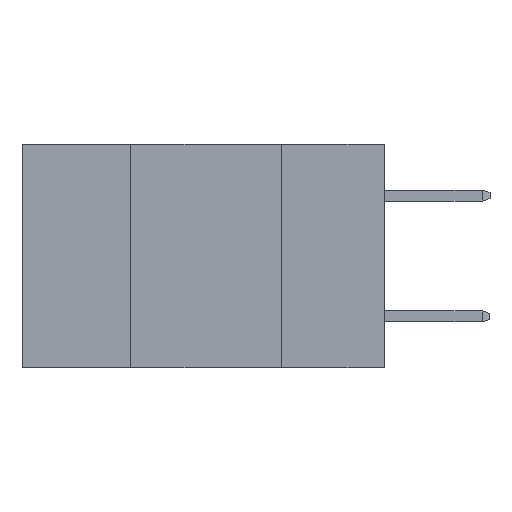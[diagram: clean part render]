
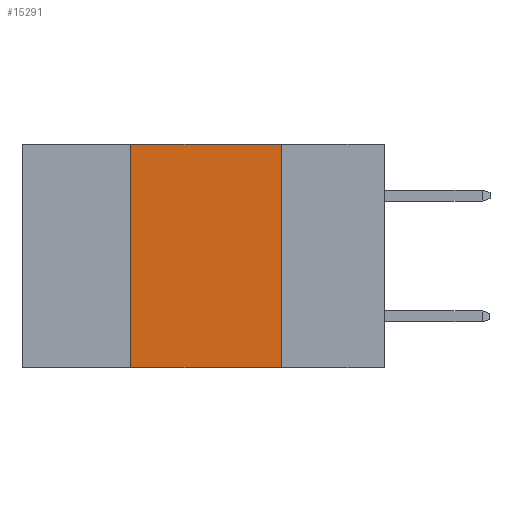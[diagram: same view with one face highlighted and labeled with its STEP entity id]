
A CAD part, left-side view. The second image highlights one B-rep face of the part: STEP entity #15291.
In plain terms, the highlighted planar face has unit normal (-1, 0, 0).
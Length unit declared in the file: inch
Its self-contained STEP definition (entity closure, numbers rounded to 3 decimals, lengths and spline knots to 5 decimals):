
#799 = EDGE_CURVE ( 'NONE', #2177, #25456, #13775, .T. ) ;
#2110 = CARTESIAN_POINT ( 'NONE',  ( 0., 0.42, 0. ) ) ;
#2177 = VERTEX_POINT ( 'NONE', #5522 ) ;
#2531 = PLANE ( 'NONE',  #17912 ) ;
#3132 = VERTEX_POINT ( 'NONE', #2110 ) ;
#3241 = EDGE_LOOP ( 'NONE', ( #24996, #9982, #10603, #21034 ) ) ;
#5432 = LINE ( 'NONE', #9356, #25142 ) ;
#5436 = DIRECTION ( 'NONE',  ( 0., 0., -1. ) ) ;
#5522 = CARTESIAN_POINT ( 'NONE',  ( 0., 0.17, 0. ) ) ;
#5713 = VERTEX_POINT ( 'NONE', #22207 ) ;
#5851 = CARTESIAN_POINT ( 'NONE',  ( 0., 0.17, 0. ) ) ;
#8556 = DIRECTION ( 'NONE',  ( 1., 0., 0. ) ) ;
#9356 = CARTESIAN_POINT ( 'NONE',  ( 0., 0.6, -0.37 ) ) ;
#9982 = ORIENTED_EDGE ( 'NONE', *, *, #11830, .F. ) ;
#10603 = ORIENTED_EDGE ( 'NONE', *, *, #13320, .F. ) ;
#10681 = EDGE_CURVE ( 'NONE', #5713, #25456, #5432, .T. ) ;
#10781 = DIRECTION ( 'NONE',  ( 0., -1., 0. ) ) ;
#11830 = EDGE_CURVE ( 'NONE', #3132, #2177, #13742, .T. ) ;
#12364 = DIRECTION ( 'NONE',  ( 0., 0., 1. ) ) ;
#13320 = EDGE_CURVE ( 'NONE', #5713, #3132, #17967, .T. ) ;
#13742 = LINE ( 'NONE', #24451, #24132 ) ;
#13775 = LINE ( 'NONE', #5851, #23907 ) ;
#14858 = FACE_OUTER_BOUND ( 'NONE', #3241, .T. ) ;
#15291 = ADVANCED_FACE ( 'NONE', ( #14858 ), #2531, .F. ) ;
#15949 = CARTESIAN_POINT ( 'NONE',  ( 0., 0.17, -0.37 ) ) ;
#17912 = AXIS2_PLACEMENT_3D ( 'NONE', #20333, #8556, #22293 ) ;
#17967 = LINE ( 'NONE', #24065, #23742 ) ;
#20333 = CARTESIAN_POINT ( 'NONE',  ( 0., 0.6, 0. ) ) ;
#21034 = ORIENTED_EDGE ( 'NONE', *, *, #10681, .T. ) ;
#22207 = CARTESIAN_POINT ( 'NONE',  ( 0., 0.42, -0.37 ) ) ;
#22293 = DIRECTION ( 'NONE',  ( 0., 0., -1. ) ) ;
#23742 = VECTOR ( 'NONE', #12364, 39.37008 ) ;
#23907 = VECTOR ( 'NONE', #5436, 39.37008 ) ;
#24065 = CARTESIAN_POINT ( 'NONE',  ( 0., 0.42, 0. ) ) ;
#24132 = VECTOR ( 'NONE', #10781, 39.37008 ) ;
#24451 = CARTESIAN_POINT ( 'NONE',  ( 0., 0.6, 0. ) ) ;
#24996 = ORIENTED_EDGE ( 'NONE', *, *, #799, .F. ) ;
#25035 = DIRECTION ( 'NONE',  ( 0., -1., 0. ) ) ;
#25142 = VECTOR ( 'NONE', #25035, 39.37008 ) ;
#25456 = VERTEX_POINT ( 'NONE', #15949 ) ;
